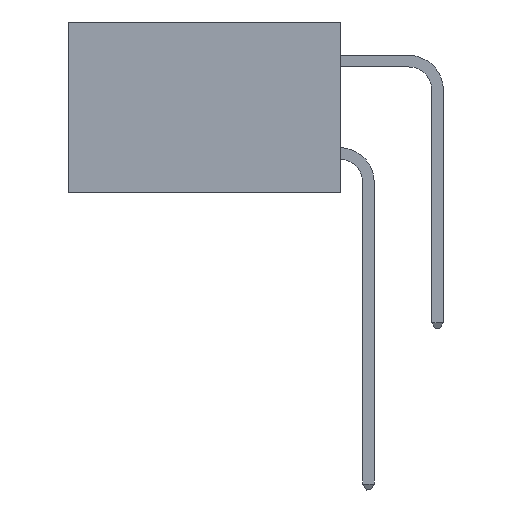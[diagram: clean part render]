
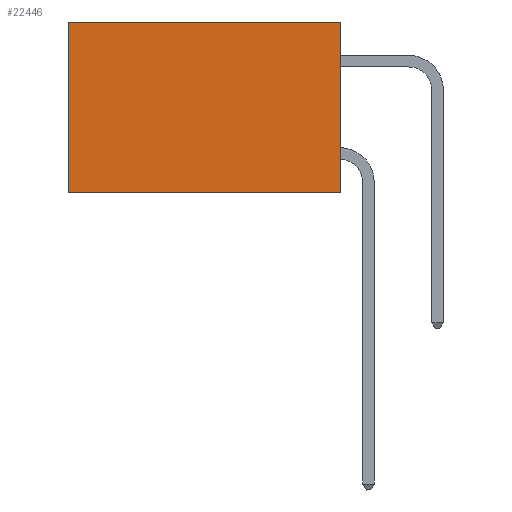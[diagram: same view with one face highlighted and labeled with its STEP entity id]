
A CAD part, left-side view. The second image highlights one B-rep face of the part: STEP entity #22446.
In plain terms, the highlighted planar face has unit normal (-1, 0, 0).
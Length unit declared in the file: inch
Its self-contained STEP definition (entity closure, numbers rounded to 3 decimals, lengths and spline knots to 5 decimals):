
#1092 = FACE_OUTER_BOUND ( 'NONE', #26773, .T. ) ;
#2599 = DIRECTION ( 'NONE',  ( 1., 0., 0. ) ) ;
#4421 = LINE ( 'NONE', #34866, #33688 ) ;
#5469 = CARTESIAN_POINT ( 'NONE',  ( 0.277, 0.59, -0.37 ) ) ;
#7022 = ORIENTED_EDGE ( 'NONE', *, *, #7447, .F. ) ;
#7447 = EDGE_CURVE ( 'NONE', #11909, #16841, #34026, .T. ) ;
#7937 = VERTEX_POINT ( 'NONE', #9510 ) ;
#9510 = CARTESIAN_POINT ( 'NONE',  ( 0.277, 0.59, 0. ) ) ;
#11909 = VERTEX_POINT ( 'NONE', #19958 ) ;
#12336 = DIRECTION ( 'NONE',  ( 0., 1., 0. ) ) ;
#13354 = VECTOR ( 'NONE', #35201, 39.37008 ) ;
#15619 = ORIENTED_EDGE ( 'NONE', *, *, #25246, .T. ) ;
#16508 = ORIENTED_EDGE ( 'NONE', *, *, #28013, .F. ) ;
#16841 = VERTEX_POINT ( 'NONE', #21327 ) ;
#17649 = CARTESIAN_POINT ( 'NONE',  ( 0.277, 0., 0. ) ) ;
#17714 = VERTEX_POINT ( 'NONE', #17649 ) ;
#19572 = CARTESIAN_POINT ( 'NONE',  ( 0.277, 0., -0.37 ) ) ;
#19958 = CARTESIAN_POINT ( 'NONE',  ( 0.277, 0., -0.37 ) ) ;
#20001 = LINE ( 'NONE', #29550, #13354 ) ;
#20826 = VECTOR ( 'NONE', #22469, 39.37008 ) ;
#21327 = CARTESIAN_POINT ( 'NONE',  ( 0.277, 0.59, -0.37 ) ) ;
#22192 = CARTESIAN_POINT ( 'NONE',  ( 0.277, 0., -0.37 ) ) ;
#22446 = ADVANCED_FACE ( 'NONE', ( #1092 ), #36377, .F. ) ;
#22447 = DIRECTION ( 'NONE',  ( 0., 0., -1. ) ) ;
#22469 = DIRECTION ( 'NONE',  ( 0., 0., -1. ) ) ;
#23743 = DIRECTION ( 'NONE',  ( 0., 1., 0. ) ) ;
#25214 = ORIENTED_EDGE ( 'NONE', *, *, #29376, .T. ) ;
#25246 = EDGE_CURVE ( 'NONE', #7937, #16841, #28379, .T. ) ;
#26773 = EDGE_LOOP ( 'NONE', ( #15619, #7022, #16508, #25214 ) ) ;
#27432 = VECTOR ( 'NONE', #23743, 39.37008 ) ;
#28013 = EDGE_CURVE ( 'NONE', #17714, #11909, #20001, .T. ) ;
#28379 = LINE ( 'NONE', #5469, #20826 ) ;
#29376 = EDGE_CURVE ( 'NONE', #17714, #7937, #4421, .T. ) ;
#29550 = CARTESIAN_POINT ( 'NONE',  ( 0.277, 0., -0.37 ) ) ;
#33688 = VECTOR ( 'NONE', #12336, 39.37008 ) ;
#34026 = LINE ( 'NONE', #22192, #27432 ) ;
#34866 = CARTESIAN_POINT ( 'NONE',  ( 0.277, 0., 0. ) ) ;
#35141 = AXIS2_PLACEMENT_3D ( 'NONE', #19572, #2599, #22447 ) ;
#35201 = DIRECTION ( 'NONE',  ( 0., 0., -1. ) ) ;
#36377 = PLANE ( 'NONE',  #35141 ) ;
